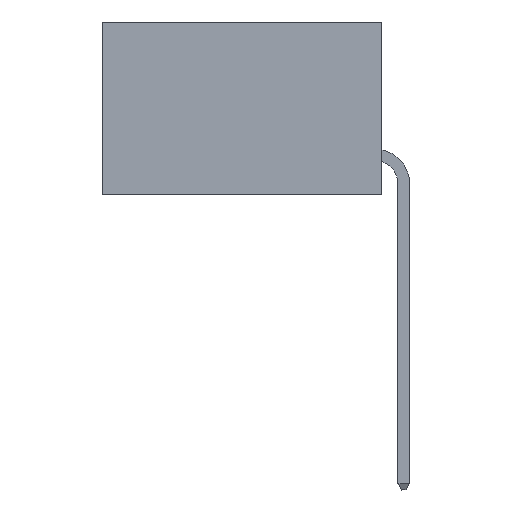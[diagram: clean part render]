
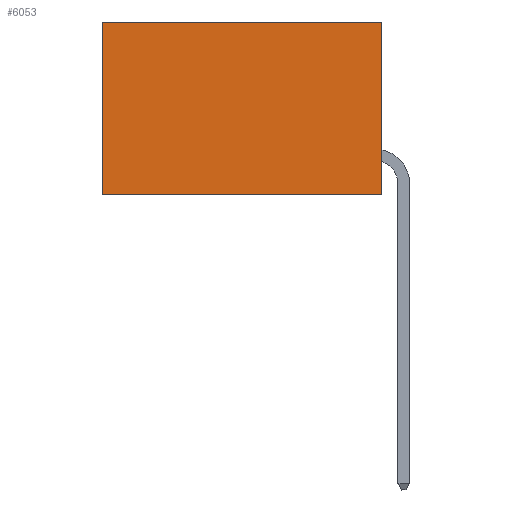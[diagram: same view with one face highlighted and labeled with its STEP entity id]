
A CAD part, left-side view. The second image highlights one B-rep face of the part: STEP entity #6053.
In plain terms, the highlighted planar face has unit normal (-1, 0, 0).
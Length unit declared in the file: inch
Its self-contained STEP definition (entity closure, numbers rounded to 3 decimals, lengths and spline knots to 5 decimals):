
#776 = LINE ( 'NONE', #22556, #10374 ) ;
#1476 = DIRECTION ( 'NONE',  ( 0., 0., -1. ) ) ;
#2542 = VERTEX_POINT ( 'NONE', #17593 ) ;
#2873 = ORIENTED_EDGE ( 'NONE', *, *, #24782, .T. ) ;
#3104 = EDGE_CURVE ( 'NONE', #9889, #22642, #776, .T. ) ;
#3581 = DIRECTION ( 'NONE',  ( 1., 0., 0. ) ) ;
#5797 = CARTESIAN_POINT ( 'NONE',  ( 0.2875, 0.6, -0.37 ) ) ;
#6053 = ADVANCED_FACE ( 'NONE', ( #10434 ), #19738, .F. ) ;
#6357 = DIRECTION ( 'NONE',  ( 0., 1., 0. ) ) ;
#7902 = CARTESIAN_POINT ( 'NONE',  ( 0.2875, 0.6, 0. ) ) ;
#8210 = CARTESIAN_POINT ( 'NONE',  ( 0.2875, 0., -0.37 ) ) ;
#8361 = EDGE_CURVE ( 'NONE', #2542, #12115, #24699, .T. ) ;
#9212 = DIRECTION ( 'NONE',  ( 0., 1., 0. ) ) ;
#9889 = VERTEX_POINT ( 'NONE', #8210 ) ;
#10277 = EDGE_LOOP ( 'NONE', ( #2873, #13735, #19908, #12763 ) ) ;
#10374 = VECTOR ( 'NONE', #6357, 39.37008 ) ;
#10434 = FACE_OUTER_BOUND ( 'NONE', #10277, .T. ) ;
#10740 = DIRECTION ( 'NONE',  ( 0., 0., -1. ) ) ;
#11652 = CARTESIAN_POINT ( 'NONE',  ( 0.2875, 0., 0. ) ) ;
#11659 = VECTOR ( 'NONE', #10740, 39.37008 ) ;
#12115 = VERTEX_POINT ( 'NONE', #7902 ) ;
#12689 = EDGE_CURVE ( 'NONE', #2542, #9889, #17069, .T. ) ;
#12704 = CARTESIAN_POINT ( 'NONE',  ( 0.2875, 0., 0. ) ) ;
#12763 = ORIENTED_EDGE ( 'NONE', *, *, #8361, .T. ) ;
#13735 = ORIENTED_EDGE ( 'NONE', *, *, #3104, .F. ) ;
#15150 = LINE ( 'NONE', #21495, #24744 ) ;
#17031 = VECTOR ( 'NONE', #9212, 39.37008 ) ;
#17069 = LINE ( 'NONE', #12704, #11659 ) ;
#17593 = CARTESIAN_POINT ( 'NONE',  ( 0.2875, 0., 0. ) ) ;
#19357 = DIRECTION ( 'NONE',  ( 0., 0., -1. ) ) ;
#19476 = AXIS2_PLACEMENT_3D ( 'NONE', #11652, #3581, #1476 ) ;
#19577 = CARTESIAN_POINT ( 'NONE',  ( 0.2875, 0., 0. ) ) ;
#19738 = PLANE ( 'NONE',  #19476 ) ;
#19908 = ORIENTED_EDGE ( 'NONE', *, *, #12689, .F. ) ;
#21495 = CARTESIAN_POINT ( 'NONE',  ( 0.2875, 0.6, 0. ) ) ;
#22556 = CARTESIAN_POINT ( 'NONE',  ( 0.2875, 0., -0.37 ) ) ;
#22642 = VERTEX_POINT ( 'NONE', #5797 ) ;
#24699 = LINE ( 'NONE', #19577, #17031 ) ;
#24744 = VECTOR ( 'NONE', #19357, 39.37008 ) ;
#24782 = EDGE_CURVE ( 'NONE', #12115, #22642, #15150, .T. ) ;
